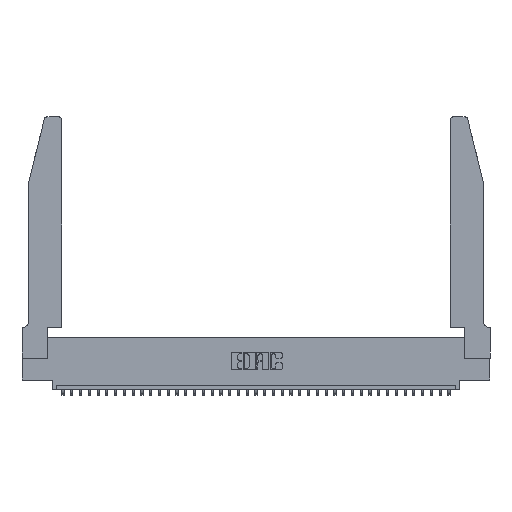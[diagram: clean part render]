
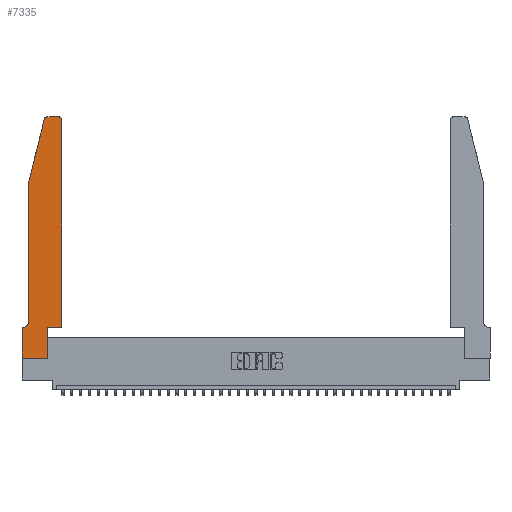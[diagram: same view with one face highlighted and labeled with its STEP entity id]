
A CAD part, top view. The second image highlights one B-rep face of the part: STEP entity #7335.
In plain terms, the highlighted planar face has unit normal (0, 0, 1).
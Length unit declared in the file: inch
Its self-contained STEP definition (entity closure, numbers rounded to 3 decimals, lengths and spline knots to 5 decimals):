
#53 = DIRECTION ( 'NONE',  ( 1., 0., 0. ) ) ;
#94 = ORIENTED_EDGE ( 'NONE', *, *, #22205, .T. ) ;
#254 = CARTESIAN_POINT ( 'NONE',  ( 0.4505, 2.72, 0.37 ) ) ;
#466 = DIRECTION ( 'NONE',  ( 1., 0., 0. ) ) ;
#480 = EDGE_CURVE ( 'NONE', #2369, #15092, #18701, .T. ) ;
#834 = VERTEX_POINT ( 'NONE', #29952 ) ;
#876 = VERTEX_POINT ( 'NONE', #254 ) ;
#1015 = CARTESIAN_POINT ( 'NONE',  ( 0.25487, 2.72718, 0.37 ) ) ;
#1699 = CARTESIAN_POINT ( 'NONE',  ( 0.4205, 2.72, 0.37 ) ) ;
#2019 = LINE ( 'NONE', #8984, #14560 ) ;
#2369 = VERTEX_POINT ( 'NONE', #5284 ) ;
#3024 = VERTEX_POINT ( 'NONE', #31526 ) ;
#3088 = CARTESIAN_POINT ( 'NONE',  ( 0., 0., 0.37 ) ) ;
#3423 = LINE ( 'NONE', #3088, #29066 ) ;
#3578 = DIRECTION ( 'NONE',  ( 1., 0., 0. ) ) ;
#4198 = CARTESIAN_POINT ( 'NONE',  ( 0., 0.35, 0.37 ) ) ;
#4247 = VECTOR ( 'NONE', #26698, 39.37008 ) ;
#5284 = CARTESIAN_POINT ( 'NONE',  ( 0.0055, 0.35, 0.37 ) ) ;
#5341 = EDGE_CURVE ( 'NONE', #12922, #876, #32678, .T. ) ;
#5825 = CARTESIAN_POINT ( 'NONE',  ( 0.0755, 0.35, 0.37 ) ) ;
#6410 = LINE ( 'NONE', #34295, #29284 ) ;
#7196 = ORIENTED_EDGE ( 'NONE', *, *, #20721, .T. ) ;
#7335 = ADVANCED_FACE ( 'NONE', ( #26517 ), #32894, .T. ) ;
#8767 = CIRCLE ( 'NONE', #9859, 0.03 ) ;
#8984 = CARTESIAN_POINT ( 'NONE',  ( 0.0755, 2., 0.37 ) ) ;
#9259 = DIRECTION ( 'NONE',  ( 0., -1., 0. ) ) ;
#9391 = CARTESIAN_POINT ( 'NONE',  ( 0.284, 2.72, 0.37 ) ) ;
#9562 = LINE ( 'NONE', #35149, #34246 ) ;
#9859 = AXIS2_PLACEMENT_3D ( 'NONE', #9391, #24106, #3578 ) ;
#10416 = DIRECTION ( 'NONE',  ( 0., 1., 0. ) ) ;
#11011 = AXIS2_PLACEMENT_3D ( 'NONE', #29602, #11776, #20849 ) ;
#11776 = DIRECTION ( 'NONE',  ( 0., 0., 1. ) ) ;
#12121 = LINE ( 'NONE', #34379, #4247 ) ;
#12282 = VERTEX_POINT ( 'NONE', #20715 ) ;
#12549 = EDGE_CURVE ( 'NONE', #36545, #3024, #12121, .T. ) ;
#12833 = DIRECTION ( 'NONE',  ( -1., 0., 0. ) ) ;
#12922 = VERTEX_POINT ( 'NONE', #27473 ) ;
#14481 = CIRCLE ( 'NONE', #29950, 0.03 ) ;
#14560 = VECTOR ( 'NONE', #29800, 39.37008 ) ;
#14753 = ORIENTED_EDGE ( 'NONE', *, *, #31103, .T. ) ;
#15035 = EDGE_CURVE ( 'NONE', #28530, #12922, #9562, .T. ) ;
#15043 = CARTESIAN_POINT ( 'NONE',  ( 0., 0., 0.37 ) ) ;
#15092 = VERTEX_POINT ( 'NONE', #4198 ) ;
#15947 = DIRECTION ( 'NONE',  ( -1., 0., 0. ) ) ;
#16875 = DIRECTION ( 'NONE',  ( 0., 0., 1. ) ) ;
#17798 = VERTEX_POINT ( 'NONE', #21774 ) ;
#18701 = LINE ( 'NONE', #5825, #30341 ) ;
#18964 = DIRECTION ( 'NONE',  ( -1., 0., 0. ) ) ;
#19850 = VERTEX_POINT ( 'NONE', #31086 ) ;
#20715 = CARTESIAN_POINT ( 'NONE',  ( 0.0755, 0.42, 0.37 ) ) ;
#20721 = EDGE_CURVE ( 'NONE', #17798, #25306, #32578, .T. ) ;
#20822 = ORIENTED_EDGE ( 'NONE', *, *, #5341, .T. ) ;
#20849 = DIRECTION ( 'NONE',  ( 1., 0., 0. ) ) ;
#21774 = CARTESIAN_POINT ( 'NONE',  ( 0.4205, 2.75, 0.37 ) ) ;
#22123 = ORIENTED_EDGE ( 'NONE', *, *, #30236, .T. ) ;
#22205 = EDGE_CURVE ( 'NONE', #25306, #36545, #8767, .T. ) ;
#22226 = CARTESIAN_POINT ( 'NONE',  ( 0.2865, 0.35, 0.37 ) ) ;
#23724 = EDGE_CURVE ( 'NONE', #12282, #2369, #24005, .T. ) ;
#24005 = CIRCLE ( 'NONE', #28662, 0.07 ) ;
#24106 = DIRECTION ( 'NONE',  ( 0., 0., 1. ) ) ;
#24305 = EDGE_LOOP ( 'NONE', ( #7196, #94, #33213, #22123, #29408, #36720, #27139, #29091, #35752, #34006, #20822, #14753 ) ) ;
#25108 = DIRECTION ( 'NONE',  ( 0., 1., 0. ) ) ;
#25306 = VERTEX_POINT ( 'NONE', #25859 ) ;
#25859 = CARTESIAN_POINT ( 'NONE',  ( 0.284, 2.75, 0.37 ) ) ;
#26517 = FACE_OUTER_BOUND ( 'NONE', #24305, .T. ) ;
#26698 = DIRECTION ( 'NONE',  ( -0.239, -0.971, 0. ) ) ;
#27139 = ORIENTED_EDGE ( 'NONE', *, *, #29569, .T. ) ;
#27473 = CARTESIAN_POINT ( 'NONE',  ( 0.4505, 0.35, 0.37 ) ) ;
#28530 = VERTEX_POINT ( 'NONE', #22226 ) ;
#28662 = AXIS2_PLACEMENT_3D ( 'NONE', #33743, #34147, #18964 ) ;
#28841 = CARTESIAN_POINT ( 'NONE',  ( 0.4505, 0.35, 0.37 ) ) ;
#29066 = VECTOR ( 'NONE', #9259, 39.37008 ) ;
#29091 = ORIENTED_EDGE ( 'NONE', *, *, #34646, .T. ) ;
#29284 = VECTOR ( 'NONE', #25108, 39.37008 ) ;
#29408 = ORIENTED_EDGE ( 'NONE', *, *, #23724, .T. ) ;
#29569 = EDGE_CURVE ( 'NONE', #15092, #834, #3423, .T. ) ;
#29602 = CARTESIAN_POINT ( 'NONE',  ( 0., 0.35, 0.37 ) ) ;
#29605 = VECTOR ( 'NONE', #53, 39.37008 ) ;
#29800 = DIRECTION ( 'NONE',  ( 0., -1., 0. ) ) ;
#29950 = AXIS2_PLACEMENT_3D ( 'NONE', #1699, #16875, #37668 ) ;
#29952 = CARTESIAN_POINT ( 'NONE',  ( 0., 0., 0.37 ) ) ;
#30236 = EDGE_CURVE ( 'NONE', #3024, #12282, #2019, .T. ) ;
#30341 = VECTOR ( 'NONE', #12833, 39.37008 ) ;
#31086 = CARTESIAN_POINT ( 'NONE',  ( 0.2865, 0., 0.37 ) ) ;
#31103 = EDGE_CURVE ( 'NONE', #876, #17798, #14481, .T. ) ;
#31301 = VECTOR ( 'NONE', #10416, 39.37008 ) ;
#31526 = CARTESIAN_POINT ( 'NONE',  ( 0.0755, 2., 0.37 ) ) ;
#32558 = EDGE_CURVE ( 'NONE', #19850, #28530, #6410, .T. ) ;
#32578 = LINE ( 'NONE', #36858, #33941 ) ;
#32678 = LINE ( 'NONE', #28841, #31301 ) ;
#32894 = PLANE ( 'NONE',  #11011 ) ;
#33213 = ORIENTED_EDGE ( 'NONE', *, *, #12549, .T. ) ;
#33743 = CARTESIAN_POINT ( 'NONE',  ( 0.0055, 0.42, 0.37 ) ) ;
#33941 = VECTOR ( 'NONE', #15947, 39.37008 ) ;
#34006 = ORIENTED_EDGE ( 'NONE', *, *, #15035, .T. ) ;
#34147 = DIRECTION ( 'NONE',  ( 0., 0., -1. ) ) ;
#34246 = VECTOR ( 'NONE', #466, 39.37008 ) ;
#34295 = CARTESIAN_POINT ( 'NONE',  ( 0.2865, 0.35, 0.37 ) ) ;
#34379 = CARTESIAN_POINT ( 'NONE',  ( 0.0755, 2., 0.37 ) ) ;
#34646 = EDGE_CURVE ( 'NONE', #834, #19850, #37483, .T. ) ;
#35149 = CARTESIAN_POINT ( 'NONE',  ( 0.4505, 0.35, 0.37 ) ) ;
#35752 = ORIENTED_EDGE ( 'NONE', *, *, #32558, .T. ) ;
#36545 = VERTEX_POINT ( 'NONE', #1015 ) ;
#36720 = ORIENTED_EDGE ( 'NONE', *, *, #480, .T. ) ;
#36858 = CARTESIAN_POINT ( 'NONE',  ( 0.2605, 2.75, 0.37 ) ) ;
#37483 = LINE ( 'NONE', #15043, #29605 ) ;
#37668 = DIRECTION ( 'NONE',  ( 1., 0., 0. ) ) ;
